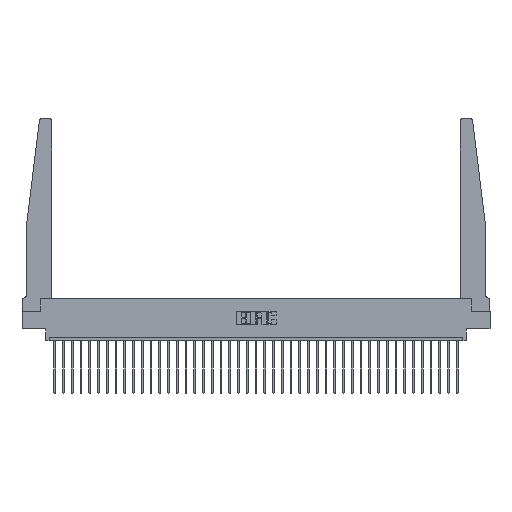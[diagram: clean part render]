
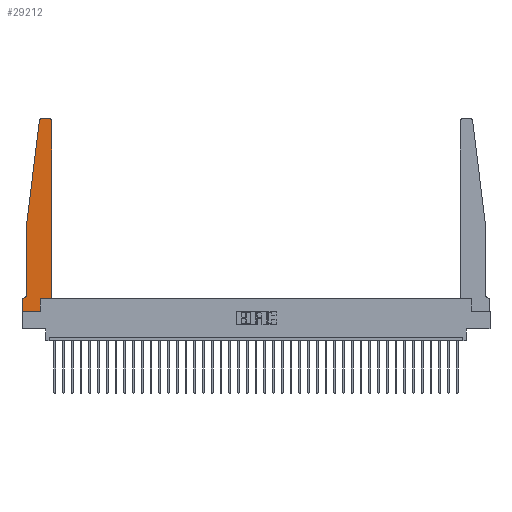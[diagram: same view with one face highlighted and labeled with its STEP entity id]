
A CAD part, top view. The second image highlights one B-rep face of the part: STEP entity #29212.
In plain terms, the highlighted planar face has unit normal (0, 0, 1).
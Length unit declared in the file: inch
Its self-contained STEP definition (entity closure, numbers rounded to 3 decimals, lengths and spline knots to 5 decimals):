
#312 = ORIENTED_EDGE ( 'NONE', *, *, #21768, .T. ) ;
#558 = ORIENTED_EDGE ( 'NONE', *, *, #30867, .T. ) ;
#657 = CARTESIAN_POINT ( 'NONE',  ( 0.2605, 0.18, 0.37 ) ) ;
#825 = ORIENTED_EDGE ( 'NONE', *, *, #32741, .T. ) ;
#1141 = VERTEX_POINT ( 'NONE', #6568 ) ;
#2026 = AXIS2_PLACEMENT_3D ( 'NONE', #11763, #27644, #20054 ) ;
#2665 = EDGE_CURVE ( 'NONE', #18798, #2958, #17938, .T. ) ;
#2746 = ORIENTED_EDGE ( 'NONE', *, *, #2665, .T. ) ;
#2958 = VERTEX_POINT ( 'NONE', #10347 ) ;
#3068 = VECTOR ( 'NONE', #7237, 39.37008 ) ;
#3348 = ORIENTED_EDGE ( 'NONE', *, *, #22643, .T. ) ;
#3881 = VECTOR ( 'NONE', #14566, 39.37008 ) ;
#4190 = CARTESIAN_POINT ( 'NONE',  ( 0.065, 1.25, 0.37 ) ) ;
#4313 = DIRECTION ( 'NONE',  ( 0., -1., 0. ) ) ;
#4446 = EDGE_CURVE ( 'NONE', #1141, #16666, #8533, .T. ) ;
#4681 = DIRECTION ( 'NONE',  ( 0., 0., -1. ) ) ;
#4825 = DIRECTION ( 'NONE',  ( 1., 0., 0. ) ) ;
#5724 = EDGE_CURVE ( 'NONE', #2958, #32433, #23902, .T. ) ;
#5823 = AXIS2_PLACEMENT_3D ( 'NONE', #18809, #24041, #8135 ) ;
#5913 = VERTEX_POINT ( 'NONE', #657 ) ;
#6035 = VERTEX_POINT ( 'NONE', #21449 ) ;
#6249 = VECTOR ( 'NONE', #14631, 39.37008 ) ;
#6257 = CARTESIAN_POINT ( 'NONE',  ( 0.425, 2.72, 0.37 ) ) ;
#6362 = CIRCLE ( 'NONE', #11499, 0.03 ) ;
#6500 = PLANE ( 'NONE',  #2026 ) ;
#6568 = CARTESIAN_POINT ( 'NONE',  ( 0.425, 0.18, 0.37 ) ) ;
#6685 = CARTESIAN_POINT ( 'NONE',  ( 0.27653, 2.75, 0.37 ) ) ;
#7075 = CARTESIAN_POINT ( 'NONE',  ( 0.25, 2.75, 0.37 ) ) ;
#7237 = DIRECTION ( 'NONE',  ( -1., 0., 0. ) ) ;
#7835 = DIRECTION ( 'NONE',  ( 0., 1., 0. ) ) ;
#8135 = DIRECTION ( 'NONE',  ( 1., 0., 0. ) ) ;
#8533 = LINE ( 'NONE', #21307, #27976 ) ;
#8597 = ORIENTED_EDGE ( 'NONE', *, *, #4446, .T. ) ;
#9080 = FACE_OUTER_BOUND ( 'NONE', #22335, .T. ) ;
#9682 = CARTESIAN_POINT ( 'NONE',  ( 0., 0., 0.37 ) ) ;
#9918 = LINE ( 'NONE', #24821, #3881 ) ;
#10086 = LINE ( 'NONE', #7075, #28705 ) ;
#10347 = CARTESIAN_POINT ( 'NONE',  ( 0.065, 0.2375, 0.37 ) ) ;
#10972 = DIRECTION ( 'NONE',  ( 0., 1., 0. ) ) ;
#11030 = ORIENTED_EDGE ( 'NONE', *, *, #19828, .T. ) ;
#11499 = AXIS2_PLACEMENT_3D ( 'NONE', #12787, #20185, #15274 ) ;
#11763 = CARTESIAN_POINT ( 'NONE',  ( 0., 0.1875, 0.37 ) ) ;
#12787 = CARTESIAN_POINT ( 'NONE',  ( 0.27653, 2.72, 0.37 ) ) ;
#12884 = VECTOR ( 'NONE', #7835, 39.37008 ) ;
#13539 = ORIENTED_EDGE ( 'NONE', *, *, #20008, .T. ) ;
#13611 = CARTESIAN_POINT ( 'NONE',  ( 0., 0., 0.37 ) ) ;
#14012 = VERTEX_POINT ( 'NONE', #6685 ) ;
#14535 = VERTEX_POINT ( 'NONE', #26607 ) ;
#14566 = DIRECTION ( 'NONE',  ( 1., 0., 0. ) ) ;
#14631 = DIRECTION ( 'NONE',  ( -0.122, -0.992, 0. ) ) ;
#14806 = CARTESIAN_POINT ( 'NONE',  ( 0.065, 0.1875, 0.37 ) ) ;
#15274 = DIRECTION ( 'NONE',  ( 1., 0., 0. ) ) ;
#16131 = LINE ( 'NONE', #23183, #12884 ) ;
#16198 = LINE ( 'NONE', #27502, #19491 ) ;
#16389 = LINE ( 'NONE', #9682, #30962 ) ;
#16666 = VERTEX_POINT ( 'NONE', #6257 ) ;
#16767 = EDGE_CURVE ( 'NONE', #14535, #26069, #16198, .T. ) ;
#16951 = AXIS2_PLACEMENT_3D ( 'NONE', #27763, #4681, #22935 ) ;
#17006 = CARTESIAN_POINT ( 'NONE',  ( 0.065, 1.25, 0.37 ) ) ;
#17938 = LINE ( 'NONE', #29319, #30064 ) ;
#18798 = VERTEX_POINT ( 'NONE', #4190 ) ;
#18809 = CARTESIAN_POINT ( 'NONE',  ( 0.395, 2.72, 0.37 ) ) ;
#19368 = ORIENTED_EDGE ( 'NONE', *, *, #26913, .T. ) ;
#19491 = VECTOR ( 'NONE', #30294, 39.37008 ) ;
#19828 = EDGE_CURVE ( 'NONE', #32433, #14535, #23764, .T. ) ;
#20008 = EDGE_CURVE ( 'NONE', #5913, #1141, #9918, .T. ) ;
#20016 = ORIENTED_EDGE ( 'NONE', *, *, #5724, .T. ) ;
#20054 = DIRECTION ( 'NONE',  ( 1., 0., 0. ) ) ;
#20185 = DIRECTION ( 'NONE',  ( 0., 0., 1. ) ) ;
#20653 = VERTEX_POINT ( 'NONE', #32752 ) ;
#21307 = CARTESIAN_POINT ( 'NONE',  ( 0.425, 0.18, 0.37 ) ) ;
#21449 = CARTESIAN_POINT ( 'NONE',  ( 0.24675, 2.72367, 0.37 ) ) ;
#21768 = EDGE_CURVE ( 'NONE', #14012, #6035, #6362, .T. ) ;
#22335 = EDGE_LOOP ( 'NONE', ( #825, #312, #28273, #2746, #20016, #11030, #26658, #3348, #19368, #13539, #8597, #558 ) ) ;
#22643 = EDGE_CURVE ( 'NONE', #26069, #24969, #16389, .T. ) ;
#22935 = DIRECTION ( 'NONE',  ( -1., 0., 0. ) ) ;
#23183 = CARTESIAN_POINT ( 'NONE',  ( 0.2605, 0.18, 0.37 ) ) ;
#23764 = LINE ( 'NONE', #14806, #3068 ) ;
#23902 = CIRCLE ( 'NONE', #16951, 0.05 ) ;
#24041 = DIRECTION ( 'NONE',  ( 0., 0., 1. ) ) ;
#24821 = CARTESIAN_POINT ( 'NONE',  ( 0.425, 0.18, 0.37 ) ) ;
#24969 = VERTEX_POINT ( 'NONE', #33199 ) ;
#25204 = DIRECTION ( 'NONE',  ( -1., 0., 0. ) ) ;
#26069 = VERTEX_POINT ( 'NONE', #13611 ) ;
#26607 = CARTESIAN_POINT ( 'NONE',  ( 0., 0.1875, 0.37 ) ) ;
#26658 = ORIENTED_EDGE ( 'NONE', *, *, #16767, .T. ) ;
#26808 = CIRCLE ( 'NONE', #5823, 0.03 ) ;
#26913 = EDGE_CURVE ( 'NONE', #24969, #5913, #16131, .T. ) ;
#27317 = LINE ( 'NONE', #17006, #6249 ) ;
#27502 = CARTESIAN_POINT ( 'NONE',  ( 0., 0., 0.37 ) ) ;
#27644 = DIRECTION ( 'NONE',  ( 0., 0., 1. ) ) ;
#27763 = CARTESIAN_POINT ( 'NONE',  ( 0.015, 0.2375, 0.37 ) ) ;
#27976 = VECTOR ( 'NONE', #10972, 39.37008 ) ;
#28273 = ORIENTED_EDGE ( 'NONE', *, *, #29544, .T. ) ;
#28705 = VECTOR ( 'NONE', #25204, 39.37008 ) ;
#29212 = ADVANCED_FACE ( 'NONE', ( #9080 ), #6500, .T. ) ;
#29319 = CARTESIAN_POINT ( 'NONE',  ( 0.065, 1.25, 0.37 ) ) ;
#29544 = EDGE_CURVE ( 'NONE', #6035, #18798, #27317, .T. ) ;
#30064 = VECTOR ( 'NONE', #4313, 39.37008 ) ;
#30294 = DIRECTION ( 'NONE',  ( 0., -1., 0. ) ) ;
#30757 = CARTESIAN_POINT ( 'NONE',  ( 0.015, 0.1875, 0.37 ) ) ;
#30867 = EDGE_CURVE ( 'NONE', #16666, #20653, #26808, .T. ) ;
#30962 = VECTOR ( 'NONE', #4825, 39.37008 ) ;
#32433 = VERTEX_POINT ( 'NONE', #30757 ) ;
#32741 = EDGE_CURVE ( 'NONE', #20653, #14012, #10086, .T. ) ;
#32752 = CARTESIAN_POINT ( 'NONE',  ( 0.395, 2.75, 0.37 ) ) ;
#33199 = CARTESIAN_POINT ( 'NONE',  ( 0.2605, 0., 0.37 ) ) ;
